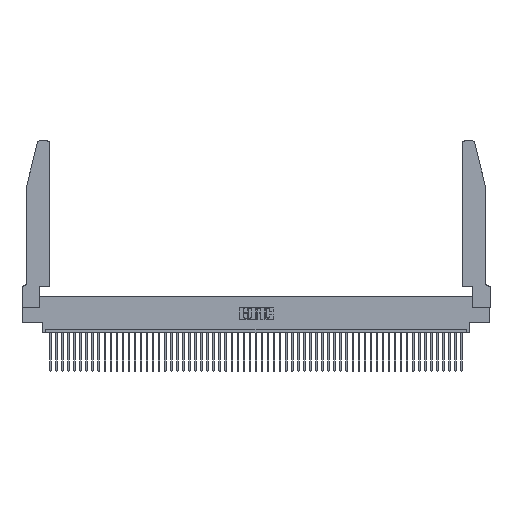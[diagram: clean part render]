
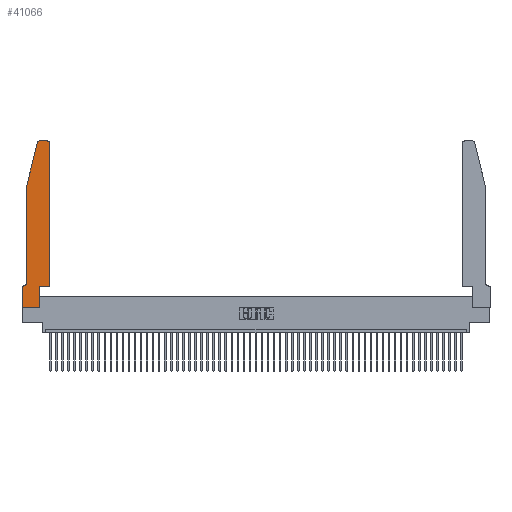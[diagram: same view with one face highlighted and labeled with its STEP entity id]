
A CAD part, top view. The second image highlights one B-rep face of the part: STEP entity #41066.
In plain terms, the highlighted planar face has unit normal (0, 0, 1).
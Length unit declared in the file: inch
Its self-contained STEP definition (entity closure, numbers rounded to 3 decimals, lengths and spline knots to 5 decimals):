
#379 = CARTESIAN_POINT ( 'NONE',  ( 0., 0.35, 0.37 ) ) ;
#389 = VERTEX_POINT ( 'NONE', #3868 ) ;
#453 = ORIENTED_EDGE ( 'NONE', *, *, #14062, .T. ) ;
#614 = ORIENTED_EDGE ( 'NONE', *, *, #5573, .T. ) ;
#729 = VERTEX_POINT ( 'NONE', #4120 ) ;
#769 = LINE ( 'NONE', #26801, #29775 ) ;
#851 = CARTESIAN_POINT ( 'NONE',  ( 0.4205, 2.72, 0.37 ) ) ;
#1338 = VERTEX_POINT ( 'NONE', #10151 ) ;
#2402 = ORIENTED_EDGE ( 'NONE', *, *, #5837, .T. ) ;
#2616 = CARTESIAN_POINT ( 'NONE',  ( 0.0755, 0.42, 0.37 ) ) ;
#3023 = DIRECTION ( 'NONE',  ( 0., 0., -1. ) ) ;
#3868 = CARTESIAN_POINT ( 'NONE',  ( 0., 0.35, 0.37 ) ) ;
#3879 = CARTESIAN_POINT ( 'NONE',  ( 0.2865, 0.35, 0.37 ) ) ;
#3884 = DIRECTION ( 'NONE',  ( 1., 0., 0. ) ) ;
#3888 = VECTOR ( 'NONE', #39051, 39.37008 ) ;
#3946 = LINE ( 'NONE', #5169, #9048 ) ;
#4086 = PLANE ( 'NONE',  #39240 ) ;
#4120 = CARTESIAN_POINT ( 'NONE',  ( 0.284, 2.75, 0.37 ) ) ;
#4933 = VECTOR ( 'NONE', #23988, 39.37008 ) ;
#5169 = CARTESIAN_POINT ( 'NONE',  ( 0.0755, 2., 0.37 ) ) ;
#5573 = EDGE_CURVE ( 'NONE', #13394, #1338, #8110, .T. ) ;
#5837 = EDGE_CURVE ( 'NONE', #16737, #13394, #769, .T. ) ;
#6309 = EDGE_LOOP ( 'NONE', ( #453, #6772, #11436, #18763, #27233, #47977, #19967, #20476, #2402, #614, #20386, #48327 ) ) ;
#6772 = ORIENTED_EDGE ( 'NONE', *, *, #33577, .T. ) ;
#7826 = CARTESIAN_POINT ( 'NONE',  ( 0., 0., 0.37 ) ) ;
#8110 = LINE ( 'NONE', #36608, #31832 ) ;
#8273 = VERTEX_POINT ( 'NONE', #14031 ) ;
#8762 = VERTEX_POINT ( 'NONE', #47135 ) ;
#9048 = VECTOR ( 'NONE', #46053, 39.37008 ) ;
#9437 = AXIS2_PLACEMENT_3D ( 'NONE', #48663, #28791, #41539 ) ;
#10029 = DIRECTION ( 'NONE',  ( -1., 0., 0. ) ) ;
#10151 = CARTESIAN_POINT ( 'NONE',  ( 0.4505, 0.35, 0.37 ) ) ;
#10204 = LINE ( 'NONE', #7826, #48129 ) ;
#10651 = EDGE_CURVE ( 'NONE', #8273, #16737, #10204, .T. ) ;
#11436 = ORIENTED_EDGE ( 'NONE', *, *, #17657, .T. ) ;
#11489 = DIRECTION ( 'NONE',  ( 0., -1., 0. ) ) ;
#11672 = LINE ( 'NONE', #39406, #3888 ) ;
#13394 = VERTEX_POINT ( 'NONE', #3879 ) ;
#14031 = CARTESIAN_POINT ( 'NONE',  ( 0., 0., 0.37 ) ) ;
#14062 = EDGE_CURVE ( 'NONE', #44913, #729, #19517, .T. ) ;
#16737 = VERTEX_POINT ( 'NONE', #40919 ) ;
#17657 = EDGE_CURVE ( 'NONE', #46412, #44538, #3946, .T. ) ;
#18763 = ORIENTED_EDGE ( 'NONE', *, *, #49573, .T. ) ;
#19517 = LINE ( 'NONE', #26341, #33535 ) ;
#19967 = ORIENTED_EDGE ( 'NONE', *, *, #49982, .T. ) ;
#20386 = ORIENTED_EDGE ( 'NONE', *, *, #38369, .T. ) ;
#20476 = ORIENTED_EDGE ( 'NONE', *, *, #10651, .T. ) ;
#20564 = DIRECTION ( 'NONE',  ( 0., 0., 1. ) ) ;
#20635 = EDGE_CURVE ( 'NONE', #48200, #389, #23656, .T. ) ;
#23582 = DIRECTION ( 'NONE',  ( 1., 0., 0. ) ) ;
#23656 = LINE ( 'NONE', #26634, #41507 ) ;
#23988 = DIRECTION ( 'NONE',  ( 0., -1., 0. ) ) ;
#24644 = CARTESIAN_POINT ( 'NONE',  ( 0.25487, 2.72718, 0.37 ) ) ;
#24864 = VECTOR ( 'NONE', #11489, 39.37008 ) ;
#26341 = CARTESIAN_POINT ( 'NONE',  ( 0.2605, 2.75, 0.37 ) ) ;
#26634 = CARTESIAN_POINT ( 'NONE',  ( 0.0755, 0.35, 0.37 ) ) ;
#26801 = CARTESIAN_POINT ( 'NONE',  ( 0.2865, 0.35, 0.37 ) ) ;
#26842 = LINE ( 'NONE', #52871, #4933 ) ;
#27233 = ORIENTED_EDGE ( 'NONE', *, *, #48924, .T. ) ;
#28791 = DIRECTION ( 'NONE',  ( 0., 0., 1. ) ) ;
#29681 = DIRECTION ( 'NONE',  ( 0., 0., 1. ) ) ;
#29719 = EDGE_CURVE ( 'NONE', #8762, #44913, #46787, .T. ) ;
#29775 = VECTOR ( 'NONE', #39135, 39.37008 ) ;
#30183 = AXIS2_PLACEMENT_3D ( 'NONE', #40148, #3023, #48776 ) ;
#31222 = VERTEX_POINT ( 'NONE', #2616 ) ;
#31832 = VECTOR ( 'NONE', #3884, 39.37008 ) ;
#33535 = VECTOR ( 'NONE', #10029, 39.37008 ) ;
#33577 = EDGE_CURVE ( 'NONE', #729, #46412, #52956, .T. ) ;
#35193 = CIRCLE ( 'NONE', #30183, 0.07 ) ;
#36608 = CARTESIAN_POINT ( 'NONE',  ( 0.4505, 0.35, 0.37 ) ) ;
#38369 = EDGE_CURVE ( 'NONE', #1338, #8762, #11672, .T. ) ;
#39017 = DIRECTION ( 'NONE',  ( 1., 0., 0. ) ) ;
#39051 = DIRECTION ( 'NONE',  ( 0., 1., 0. ) ) ;
#39124 = CARTESIAN_POINT ( 'NONE',  ( 0.0055, 0.35, 0.37 ) ) ;
#39135 = DIRECTION ( 'NONE',  ( 0., 1., 0. ) ) ;
#39240 = AXIS2_PLACEMENT_3D ( 'NONE', #379, #20564, #40998 ) ;
#39406 = CARTESIAN_POINT ( 'NONE',  ( 0.4505, 0.35, 0.37 ) ) ;
#40148 = CARTESIAN_POINT ( 'NONE',  ( 0.0055, 0.42, 0.37 ) ) ;
#40919 = CARTESIAN_POINT ( 'NONE',  ( 0.2865, 0., 0.37 ) ) ;
#40998 = DIRECTION ( 'NONE',  ( 1., 0., 0. ) ) ;
#41066 = ADVANCED_FACE ( 'NONE', ( #49970 ), #4086, .T. ) ;
#41287 = CARTESIAN_POINT ( 'NONE',  ( 0.4205, 2.75, 0.37 ) ) ;
#41507 = VECTOR ( 'NONE', #41619, 39.37008 ) ;
#41539 = DIRECTION ( 'NONE',  ( 1., 0., 0. ) ) ;
#41619 = DIRECTION ( 'NONE',  ( -1., 0., 0. ) ) ;
#44538 = VERTEX_POINT ( 'NONE', #50095 ) ;
#44616 = CARTESIAN_POINT ( 'NONE',  ( 0.0755, 2., 0.37 ) ) ;
#44913 = VERTEX_POINT ( 'NONE', #41287 ) ;
#45704 = AXIS2_PLACEMENT_3D ( 'NONE', #851, #29681, #39017 ) ;
#46053 = DIRECTION ( 'NONE',  ( -0.239, -0.971, 0. ) ) ;
#46412 = VERTEX_POINT ( 'NONE', #24644 ) ;
#46787 = CIRCLE ( 'NONE', #45704, 0.03 ) ;
#47135 = CARTESIAN_POINT ( 'NONE',  ( 0.4505, 2.72, 0.37 ) ) ;
#47977 = ORIENTED_EDGE ( 'NONE', *, *, #20635, .T. ) ;
#48129 = VECTOR ( 'NONE', #23582, 39.37008 ) ;
#48200 = VERTEX_POINT ( 'NONE', #39124 ) ;
#48327 = ORIENTED_EDGE ( 'NONE', *, *, #29719, .T. ) ;
#48663 = CARTESIAN_POINT ( 'NONE',  ( 0.284, 2.72, 0.37 ) ) ;
#48776 = DIRECTION ( 'NONE',  ( -1., 0., 0. ) ) ;
#48924 = EDGE_CURVE ( 'NONE', #31222, #48200, #35193, .T. ) ;
#49573 = EDGE_CURVE ( 'NONE', #44538, #31222, #51856, .T. ) ;
#49970 = FACE_OUTER_BOUND ( 'NONE', #6309, .T. ) ;
#49982 = EDGE_CURVE ( 'NONE', #389, #8273, #26842, .T. ) ;
#50095 = CARTESIAN_POINT ( 'NONE',  ( 0.0755, 2., 0.37 ) ) ;
#51856 = LINE ( 'NONE', #44616, #24864 ) ;
#52871 = CARTESIAN_POINT ( 'NONE',  ( 0., 0., 0.37 ) ) ;
#52956 = CIRCLE ( 'NONE', #9437, 0.03 ) ;
